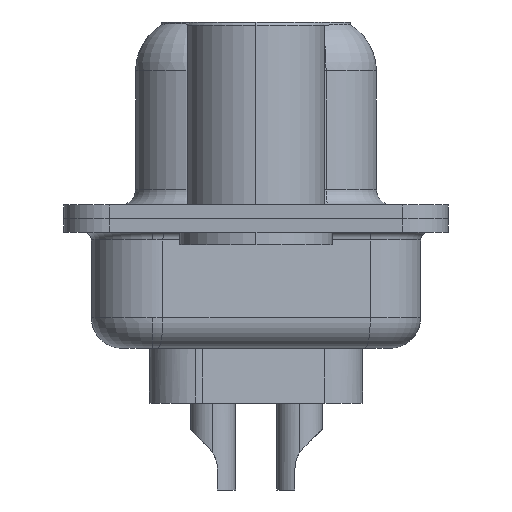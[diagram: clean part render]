
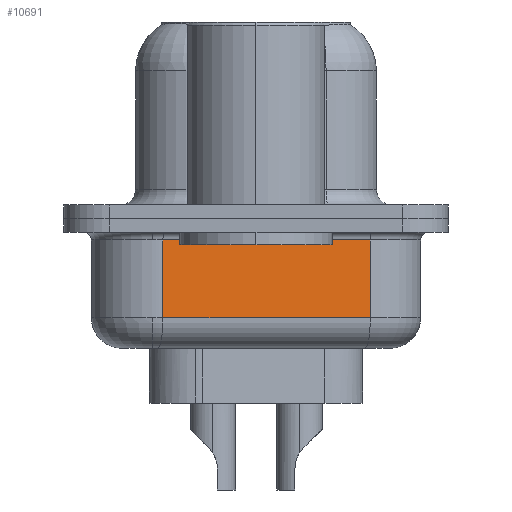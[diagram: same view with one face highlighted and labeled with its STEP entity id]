
A CAD part, left-side view. The second image highlights one B-rep face of the part: STEP entity #10691.
In plain terms, the highlighted planar face has unit normal (-0.985, -0.174, 0).
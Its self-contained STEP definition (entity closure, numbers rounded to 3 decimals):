
#1812 = VERTEX_POINT ( 'NONE', #14283 ) ;
#1939 = VECTOR ( 'NONE', #11425, 1000. ) ;
#2181 = VECTOR ( 'NONE', #14745, 1000. ) ;
#2408 = PLANE ( 'NONE',  #16880 ) ;
#2901 = VERTEX_POINT ( 'NONE', #16706 ) ;
#3291 = CARTESIAN_POINT ( 'NONE',  ( 2.875, 3.053, -4.25 ) ) ;
#3572 = CARTESIAN_POINT ( 'NONE',  ( 2.875, 3.053, -3.25 ) ) ;
#4204 = EDGE_CURVE ( 'NONE', #6625, #1812, #19099, .T. ) ;
#4382 = VERTEX_POINT ( 'NONE', #14324 ) ;
#5394 = CARTESIAN_POINT ( 'NONE',  ( 2.875, 3.053, -4.25 ) ) ;
#5499 = EDGE_LOOP ( 'NONE', ( #14154, #16890, #13080, #18843 ) ) ;
#6111 = EDGE_CURVE ( 'NONE', #1812, #2901, #12749, .T. ) ;
#6462 = CARTESIAN_POINT ( 'NONE',  ( 4.074, -3.747, -4.25 ) ) ;
#6612 = DIRECTION ( 'NONE',  ( 0., 0., 1. ) ) ;
#6625 = VERTEX_POINT ( 'NONE', #3572 ) ;
#7256 = CARTESIAN_POINT ( 'NONE',  ( 2.875, 3.053, -3.25 ) ) ;
#7775 = VECTOR ( 'NONE', #17487, 1000. ) ;
#8149 = DIRECTION ( 'NONE',  ( -0.174, 0.985, 0. ) ) ;
#8579 = EDGE_CURVE ( 'NONE', #2901, #4382, #17172, .T. ) ;
#10691 = ADVANCED_FACE ( 'NONE', ( #19188 ), #2408, .F. ) ;
#11425 = DIRECTION ( 'NONE',  ( 0., 0., 1. ) ) ;
#12530 = CARTESIAN_POINT ( 'NONE',  ( 2.875, 3.053, -0.7 ) ) ;
#12749 = LINE ( 'NONE', #6462, #1939 ) ;
#13080 = ORIENTED_EDGE ( 'NONE', *, *, #6111, .T. ) ;
#13628 = EDGE_CURVE ( 'NONE', #6625, #4382, #18868, .T. ) ;
#14154 = ORIENTED_EDGE ( 'NONE', *, *, #13628, .F. ) ;
#14283 = CARTESIAN_POINT ( 'NONE',  ( 4.074, -3.747, -3.25 ) ) ;
#14324 = CARTESIAN_POINT ( 'NONE',  ( 2.875, 3.053, -0.7 ) ) ;
#14745 = DIRECTION ( 'NONE',  ( 0.174, -0.985, 0. ) ) ;
#16593 = VECTOR ( 'NONE', #6612, 1000. ) ;
#16706 = CARTESIAN_POINT ( 'NONE',  ( 4.074, -3.747, -0.7 ) ) ;
#16880 = AXIS2_PLACEMENT_3D ( 'NONE', #5394, #19284, #8149 ) ;
#16890 = ORIENTED_EDGE ( 'NONE', *, *, #4204, .T. ) ;
#17172 = LINE ( 'NONE', #12530, #7775 ) ;
#17487 = DIRECTION ( 'NONE',  ( -0.174, 0.985, 0. ) ) ;
#18843 = ORIENTED_EDGE ( 'NONE', *, *, #8579, .T. ) ;
#18868 = LINE ( 'NONE', #3291, #16593 ) ;
#19099 = LINE ( 'NONE', #7256, #2181 ) ;
#19188 = FACE_OUTER_BOUND ( 'NONE', #5499, .T. ) ;
#19284 = DIRECTION ( 'NONE',  ( 0.985, 0.174, 0. ) ) ;
